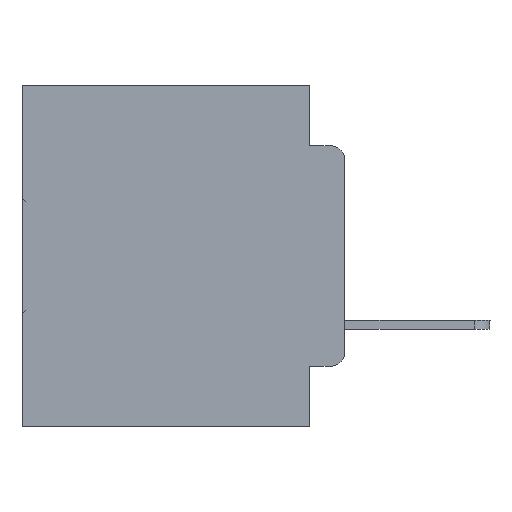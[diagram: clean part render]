
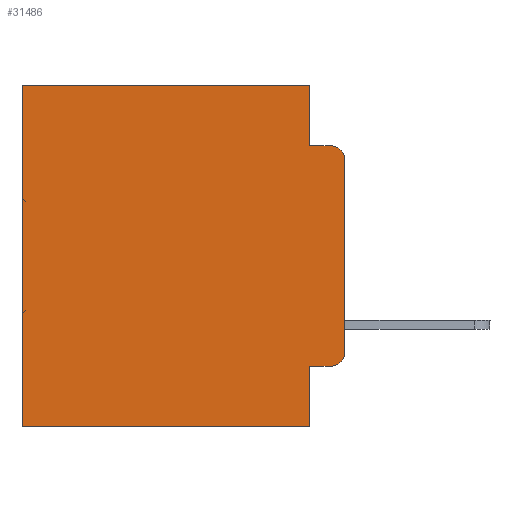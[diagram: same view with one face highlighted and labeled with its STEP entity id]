
A CAD part, left-side view. The second image highlights one B-rep face of the part: STEP entity #31486.
In plain terms, the highlighted planar face has unit normal (-1, 0, 0).
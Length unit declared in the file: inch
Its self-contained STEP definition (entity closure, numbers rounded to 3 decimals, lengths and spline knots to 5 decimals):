
#189 = LINE ( 'NONE', #17245, #16417 ) ;
#262 = CARTESIAN_POINT ( 'NONE',  ( 0.298, 0.02, -0.0885 ) ) ;
#427 = LINE ( 'NONE', #21900, #11348 ) ;
#742 = EDGE_CURVE ( 'NONE', #33050, #7578, #18662, .T. ) ;
#961 = VERTEX_POINT ( 'NONE', #8800 ) ;
#1494 = DIRECTION ( 'NONE',  ( 0., 1., 0. ) ) ;
#1799 = LINE ( 'NONE', #27691, #7045 ) ;
#1928 = DIRECTION ( 'NONE',  ( 0., 1., 0. ) ) ;
#1974 = CARTESIAN_POINT ( 'NONE',  ( 0.298, 0.051, -0.4115 ) ) ;
#2396 = EDGE_CURVE ( 'NONE', #18342, #6110, #31864, .T. ) ;
#3935 = AXIS2_PLACEMENT_3D ( 'NONE', #5899, #18579, #31313 ) ;
#4097 = VERTEX_POINT ( 'NONE', #15276 ) ;
#4248 = ORIENTED_EDGE ( 'NONE', *, *, #27983, .T. ) ;
#4803 = DIRECTION ( 'NONE',  ( 0., -1., 0. ) ) ;
#5064 = EDGE_CURVE ( 'NONE', #4097, #7578, #16314, .T. ) ;
#5899 = CARTESIAN_POINT ( 'NONE',  ( 0.298, 0., 0. ) ) ;
#6110 = VERTEX_POINT ( 'NONE', #14796 ) ;
#6852 = EDGE_CURVE ( 'NONE', #961, #23544, #427, .T. ) ;
#7045 = VECTOR ( 'NONE', #32599, 39.37008 ) ;
#7369 = DIRECTION ( 'NONE',  ( 0., 0., -1. ) ) ;
#7578 = VERTEX_POINT ( 'NONE', #32801 ) ;
#8147 = VECTOR ( 'NONE', #17374, 39.37008 ) ;
#8800 = CARTESIAN_POINT ( 'NONE',  ( 0.298, 0.051, -0.5 ) ) ;
#9218 = EDGE_CURVE ( 'NONE', #33050, #26322, #11990, .T. ) ;
#10255 = CARTESIAN_POINT ( 'NONE',  ( 0.298, 0.02, -0.1085 ) ) ;
#10876 = DIRECTION ( 'NONE',  ( 0., 0., -1. ) ) ;
#11123 = ORIENTED_EDGE ( 'NONE', *, *, #19994, .F. ) ;
#11214 = EDGE_CURVE ( 'NONE', #29818, #26322, #1799, .T. ) ;
#11348 = VECTOR ( 'NONE', #1494, 39.37008 ) ;
#11943 = AXIS2_PLACEMENT_3D ( 'NONE', #24810, #27625, #30261 ) ;
#11990 = CIRCLE ( 'NONE', #12760, 0.02 ) ;
#12237 = ORIENTED_EDGE ( 'NONE', *, *, #5064, .T. ) ;
#12385 = VECTOR ( 'NONE', #10876, 39.37008 ) ;
#12760 = AXIS2_PLACEMENT_3D ( 'NONE', #10255, #21175, #24754 ) ;
#13217 = VECTOR ( 'NONE', #4803, 39.37008 ) ;
#13477 = CARTESIAN_POINT ( 'NONE',  ( 0.298, 0.051, -0.0885 ) ) ;
#13804 = VECTOR ( 'NONE', #7369, 39.37008 ) ;
#14796 = CARTESIAN_POINT ( 'NONE',  ( 0.298, 0.473, 0. ) ) ;
#14838 = LINE ( 'NONE', #18793, #12385 ) ;
#15276 = CARTESIAN_POINT ( 'NONE',  ( 0.298, 0.02, -0.4115 ) ) ;
#15671 = EDGE_CURVE ( 'NONE', #6110, #23544, #189, .T. ) ;
#16314 = CIRCLE ( 'NONE', #11943, 0.02 ) ;
#16417 = VECTOR ( 'NONE', #17017, 39.37008 ) ;
#16449 = CARTESIAN_POINT ( 'NONE',  ( 0.298, 0.473, -0.5 ) ) ;
#17017 = DIRECTION ( 'NONE',  ( 0., 0., -1. ) ) ;
#17245 = CARTESIAN_POINT ( 'NONE',  ( 0.298, 0.473, 0. ) ) ;
#17374 = DIRECTION ( 'NONE',  ( 0., 0., -1. ) ) ;
#17910 = CARTESIAN_POINT ( 'NONE',  ( 0.298, 0., 0. ) ) ;
#18342 = VERTEX_POINT ( 'NONE', #29023 ) ;
#18579 = DIRECTION ( 'NONE',  ( 1., 0., 0. ) ) ;
#18662 = LINE ( 'NONE', #17910, #13804 ) ;
#18793 = CARTESIAN_POINT ( 'NONE',  ( 0.298, 0.051, 0. ) ) ;
#19357 = ORIENTED_EDGE ( 'NONE', *, *, #15671, .T. ) ;
#19994 = EDGE_CURVE ( 'NONE', #18342, #29818, #14838, .T. ) ;
#21175 = DIRECTION ( 'NONE',  ( -1., 0., 0. ) ) ;
#21338 = PLANE ( 'NONE',  #3935 ) ;
#21900 = CARTESIAN_POINT ( 'NONE',  ( 0.298, 0., -0.5 ) ) ;
#23544 = VERTEX_POINT ( 'NONE', #16449 ) ;
#23800 = ORIENTED_EDGE ( 'NONE', *, *, #9218, .T. ) ;
#23853 = ORIENTED_EDGE ( 'NONE', *, *, #32848, .F. ) ;
#23917 = EDGE_LOOP ( 'NONE', ( #28332, #23800, #24120, #11123, #31001, #19357, #30457, #23853, #4248, #12237 ) ) ;
#24120 = ORIENTED_EDGE ( 'NONE', *, *, #11214, .F. ) ;
#24754 = DIRECTION ( 'NONE',  ( 0., 0., -1. ) ) ;
#24810 = CARTESIAN_POINT ( 'NONE',  ( 0.298, 0.02, -0.3915 ) ) ;
#25159 = VERTEX_POINT ( 'NONE', #1974 ) ;
#25741 = CARTESIAN_POINT ( 'NONE',  ( 0.298, 0., -0.1085 ) ) ;
#26178 = VECTOR ( 'NONE', #1928, 39.37008 ) ;
#26322 = VERTEX_POINT ( 'NONE', #262 ) ;
#27095 = LINE ( 'NONE', #32695, #8147 ) ;
#27625 = DIRECTION ( 'NONE',  ( -1., 0., 0. ) ) ;
#27691 = CARTESIAN_POINT ( 'NONE',  ( 0.298, 0.051, -0.0885 ) ) ;
#27955 = CARTESIAN_POINT ( 'NONE',  ( 0.298, 0., 0. ) ) ;
#27983 = EDGE_CURVE ( 'NONE', #25159, #4097, #28535, .T. ) ;
#28332 = ORIENTED_EDGE ( 'NONE', *, *, #742, .F. ) ;
#28535 = LINE ( 'NONE', #33051, #13217 ) ;
#29023 = CARTESIAN_POINT ( 'NONE',  ( 0.298, 0.051, 0. ) ) ;
#29818 = VERTEX_POINT ( 'NONE', #13477 ) ;
#30261 = DIRECTION ( 'NONE',  ( 0., 0., -1. ) ) ;
#30457 = ORIENTED_EDGE ( 'NONE', *, *, #6852, .F. ) ;
#31001 = ORIENTED_EDGE ( 'NONE', *, *, #2396, .T. ) ;
#31213 = FACE_OUTER_BOUND ( 'NONE', #23917, .T. ) ;
#31313 = DIRECTION ( 'NONE',  ( 0., 0., -1. ) ) ;
#31486 = ADVANCED_FACE ( 'NONE', ( #31213 ), #21338, .F. ) ;
#31864 = LINE ( 'NONE', #27955, #26178 ) ;
#32599 = DIRECTION ( 'NONE',  ( 0., -1., 0. ) ) ;
#32695 = CARTESIAN_POINT ( 'NONE',  ( 0.298, 0.051, 0. ) ) ;
#32801 = CARTESIAN_POINT ( 'NONE',  ( 0.298, 0., -0.3915 ) ) ;
#32848 = EDGE_CURVE ( 'NONE', #25159, #961, #27095, .T. ) ;
#33050 = VERTEX_POINT ( 'NONE', #25741 ) ;
#33051 = CARTESIAN_POINT ( 'NONE',  ( 0.298, 0.051, -0.4115 ) ) ;
